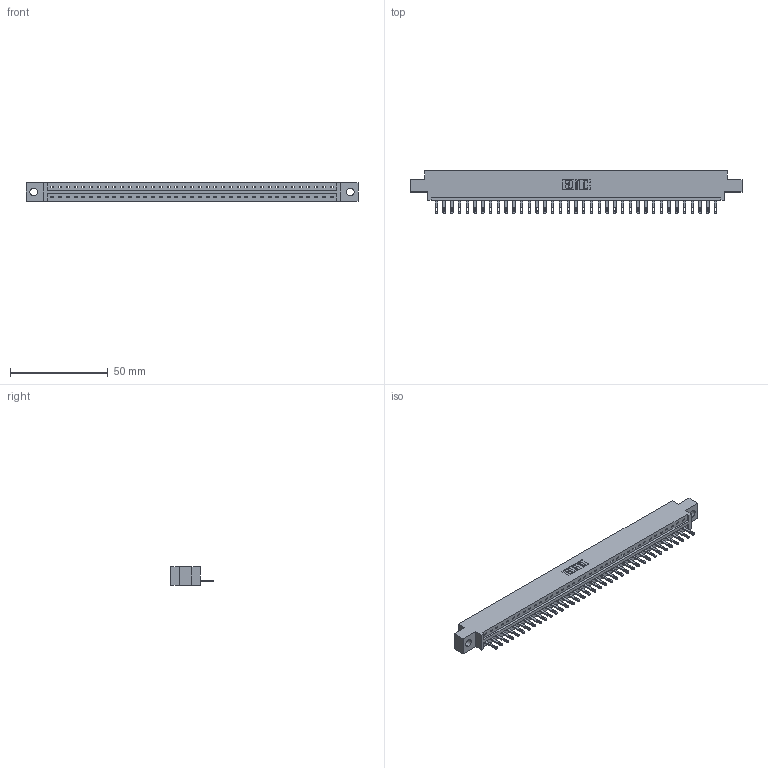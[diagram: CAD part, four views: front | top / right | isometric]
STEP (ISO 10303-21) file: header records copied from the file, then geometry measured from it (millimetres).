
FILE_DESCRIPTION (( 'STEP AP203' ), '1' );
FILE_NAME ('337-037-500-604.STEP', '2019-10-01T14:54:28', ( '' ), ( '' ), 'SwSTEP 2.0', 'SolidWorks 2016', '' );
FILE_SCHEMA (( 'CONFIG_CONTROL_DESIGN' ));
Length unit declared in the file: inch
Products named in the file (3): 345-292-001_345-293-100; 337 Part_0.170 Offset - 0.156 Dia-TH; 337-037-500-604
Assembly tree (38 placements, depth 2):
  337-037-500-604
    337 Part_0.170 Offset - 0.156 Dia-TH
    345-292-001_345-293-100  x37
Bounding box: 169.62 x 21.85 x 9.4 mm (x, y, z)
Volume: 17384.2 mm3; surface area: 17914.4 mm2
Topology: 38 solids, 38 shells, 2264 faces, 6983 edges, 4654 vertices
Faces by surface type: plane 1554, cylinder 710
Entity records: 28215 total; most frequent: CARTESIAN_POINT 4921, ORIENTED_EDGE 4894, DIRECTION 4153, EDGE_CURVE 2447, VECTOR 2315, LINE 2315, VERTEX_POINT 1630, AXIS2_PLACEMENT_3D 919
